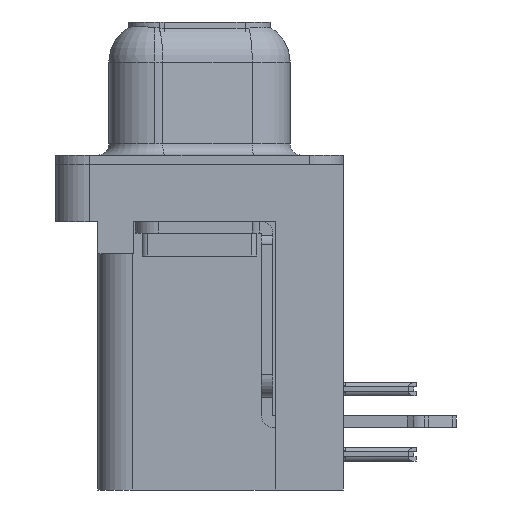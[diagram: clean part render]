
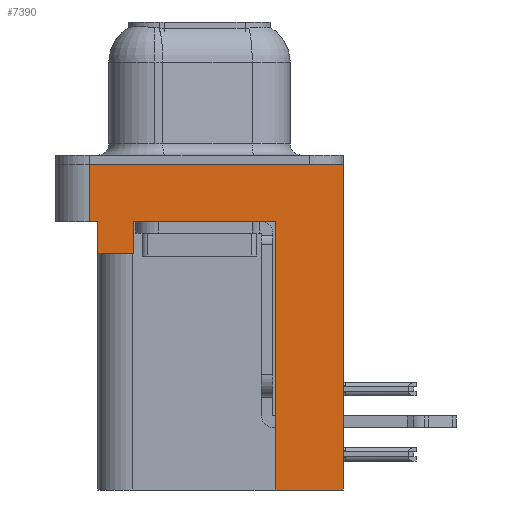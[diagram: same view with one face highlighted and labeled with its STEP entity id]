
A CAD part, left-side view. The second image highlights one B-rep face of the part: STEP entity #7390.
In plain terms, the highlighted planar face has unit normal (-1, 0, 0).
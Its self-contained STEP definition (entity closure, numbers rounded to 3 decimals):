
#158 = EDGE_CURVE ( 'NONE', #27990, #9295, #20793, .T. ) ;
#239 = DIRECTION ( 'NONE',  ( 0., 0., 1. ) ) ;
#832 = VECTOR ( 'NONE', #3790, 1000. ) ;
#1038 = CARTESIAN_POINT ( 'NONE',  ( -3., -3.295, -14.2 ) ) ;
#2468 = EDGE_CURVE ( 'NONE', #9295, #13045, #15858, .T. ) ;
#2495 = ORIENTED_EDGE ( 'NONE', *, *, #27567, .F. ) ;
#2806 = CARTESIAN_POINT ( 'NONE',  ( -3., 4.425, -3.9 ) ) ;
#2877 = EDGE_CURVE ( 'NONE', #6228, #5397, #18519, .T. ) ;
#3318 = LINE ( 'NONE', #20777, #18531 ) ;
#3460 = ORIENTED_EDGE ( 'NONE', *, *, #16261, .F. ) ;
#3790 = DIRECTION ( 'NONE',  ( 0., 0., 1. ) ) ;
#3995 = CARTESIAN_POINT ( 'NONE',  ( -3., 4.775, -2.5 ) ) ;
#5397 = VERTEX_POINT ( 'NONE', #16678 ) ;
#5488 = CARTESIAN_POINT ( 'NONE',  ( -3., 4.425, -3.9 ) ) ;
#5615 = ORIENTED_EDGE ( 'NONE', *, *, #16527, .F. ) ;
#5639 = DIRECTION ( 'NONE',  ( 0., 1., 0. ) ) ;
#6030 = FACE_OUTER_BOUND ( 'NONE', #25388, .T. ) ;
#6197 = LINE ( 'NONE', #28483, #23627 ) ;
#6228 = VERTEX_POINT ( 'NONE', #31670 ) ;
#6584 = VERTEX_POINT ( 'NONE', #1038 ) ;
#6791 = EDGE_CURVE ( 'NONE', #29066, #12842, #7085, .T. ) ;
#6821 = VERTEX_POINT ( 'NONE', #26670 ) ;
#7085 = LINE ( 'NONE', #26504, #19604 ) ;
#7390 = ADVANCED_FACE ( 'NONE', ( #6030 ), #15824, .T. ) ;
#8222 = CARTESIAN_POINT ( 'NONE',  ( -3., -3.295, -2.5 ) ) ;
#8318 = CARTESIAN_POINT ( 'NONE',  ( -3., 2.895, -2.5 ) ) ;
#8817 = VECTOR ( 'NONE', #18099, 1000. ) ;
#9210 = DIRECTION ( 'NONE',  ( 0., -1., 0. ) ) ;
#9295 = VERTEX_POINT ( 'NONE', #8318 ) ;
#9373 = CARTESIAN_POINT ( 'NONE',  ( -3., -6.275, 0. ) ) ;
#10823 = ORIENTED_EDGE ( 'NONE', *, *, #2877, .T. ) ;
#11323 = DIRECTION ( 'NONE',  ( 0., 0., 1. ) ) ;
#11765 = ORIENTED_EDGE ( 'NONE', *, *, #12088, .T. ) ;
#12088 = EDGE_CURVE ( 'NONE', #13016, #12842, #3318, .T. ) ;
#12094 = VECTOR ( 'NONE', #239, 1000. ) ;
#12842 = VERTEX_POINT ( 'NONE', #9373 ) ;
#13016 = VERTEX_POINT ( 'NONE', #17865 ) ;
#13045 = VERTEX_POINT ( 'NONE', #8222 ) ;
#13402 = DIRECTION ( 'NONE',  ( 0., 0., 1. ) ) ;
#13471 = VECTOR ( 'NONE', #13767, 1000. ) ;
#13767 = DIRECTION ( 'NONE',  ( 0., 0., 1. ) ) ;
#15824 = PLANE ( 'NONE',  #26451 ) ;
#15858 = LINE ( 'NONE', #25784, #8817 ) ;
#16261 = EDGE_CURVE ( 'NONE', #13016, #6584, #16269, .T. ) ;
#16269 = LINE ( 'NONE', #21237, #22320 ) ;
#16527 = EDGE_CURVE ( 'NONE', #6821, #5397, #24298, .T. ) ;
#16678 = CARTESIAN_POINT ( 'NONE',  ( -3., 4.425, -2.5 ) ) ;
#17070 = VECTOR ( 'NONE', #9210, 1000. ) ;
#17865 = CARTESIAN_POINT ( 'NONE',  ( -3., -6.275, -14.2 ) ) ;
#18099 = DIRECTION ( 'NONE',  ( 0., -1., 0. ) ) ;
#18519 = LINE ( 'NONE', #31342, #17070 ) ;
#18523 = DIRECTION ( 'NONE',  ( -1., 0., 0. ) ) ;
#18531 = VECTOR ( 'NONE', #25270, 1000. ) ;
#19604 = VECTOR ( 'NONE', #26024, 1000. ) ;
#20609 = EDGE_CURVE ( 'NONE', #27990, #6821, #21862, .T. ) ;
#20777 = CARTESIAN_POINT ( 'NONE',  ( -3., -6.275, -2.5 ) ) ;
#20793 = LINE ( 'NONE', #25746, #832 ) ;
#21237 = CARTESIAN_POINT ( 'NONE',  ( -3., -3.295, -14.2 ) ) ;
#21287 = ORIENTED_EDGE ( 'NONE', *, *, #158, .T. ) ;
#21304 = LINE ( 'NONE', #3995, #13471 ) ;
#21862 = LINE ( 'NONE', #5488, #23959 ) ;
#22154 = ORIENTED_EDGE ( 'NONE', *, *, #2468, .T. ) ;
#22320 = VECTOR ( 'NONE', #30695, 1000. ) ;
#23197 = CARTESIAN_POINT ( 'NONE',  ( -3., -6.275, -2.5 ) ) ;
#23627 = VECTOR ( 'NONE', #11323, 1000. ) ;
#23959 = VECTOR ( 'NONE', #5639, 1000. ) ;
#24298 = LINE ( 'NONE', #2806, #12094 ) ;
#25157 = EDGE_CURVE ( 'NONE', #6584, #13045, #6197, .T. ) ;
#25270 = DIRECTION ( 'NONE',  ( 0., 0., 1. ) ) ;
#25388 = EDGE_LOOP ( 'NONE', ( #30606, #2495, #10823, #5615, #31294, #21287, #22154, #31100, #3460, #11765 ) ) ;
#25746 = CARTESIAN_POINT ( 'NONE',  ( -3., 2.895, -3.9 ) ) ;
#25784 = CARTESIAN_POINT ( 'NONE',  ( -3., -6.275, -2.5 ) ) ;
#26024 = DIRECTION ( 'NONE',  ( 0., -1., 0. ) ) ;
#26451 = AXIS2_PLACEMENT_3D ( 'NONE', #23197, #18523, #13402 ) ;
#26504 = CARTESIAN_POINT ( 'NONE',  ( -3., -6.275, 0. ) ) ;
#26561 = CARTESIAN_POINT ( 'NONE',  ( -3., 4.775, 0. ) ) ;
#26670 = CARTESIAN_POINT ( 'NONE',  ( -3., 4.425, -3.9 ) ) ;
#27567 = EDGE_CURVE ( 'NONE', #6228, #29066, #21304, .T. ) ;
#27990 = VERTEX_POINT ( 'NONE', #28161 ) ;
#28161 = CARTESIAN_POINT ( 'NONE',  ( -3., 2.895, -3.9 ) ) ;
#28483 = CARTESIAN_POINT ( 'NONE',  ( -3., -3.295, -14.2 ) ) ;
#29066 = VERTEX_POINT ( 'NONE', #26561 ) ;
#30606 = ORIENTED_EDGE ( 'NONE', *, *, #6791, .F. ) ;
#30695 = DIRECTION ( 'NONE',  ( 0., 1., 0. ) ) ;
#31100 = ORIENTED_EDGE ( 'NONE', *, *, #25157, .F. ) ;
#31294 = ORIENTED_EDGE ( 'NONE', *, *, #20609, .F. ) ;
#31342 = CARTESIAN_POINT ( 'NONE',  ( -3., -6.275, -2.5 ) ) ;
#31670 = CARTESIAN_POINT ( 'NONE',  ( -3., 4.775, -2.5 ) ) ;
